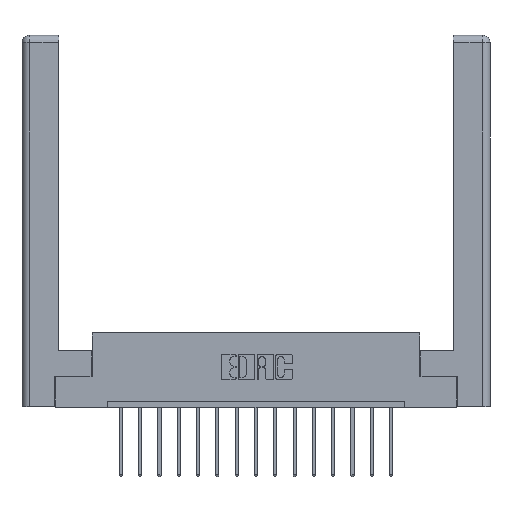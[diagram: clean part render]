
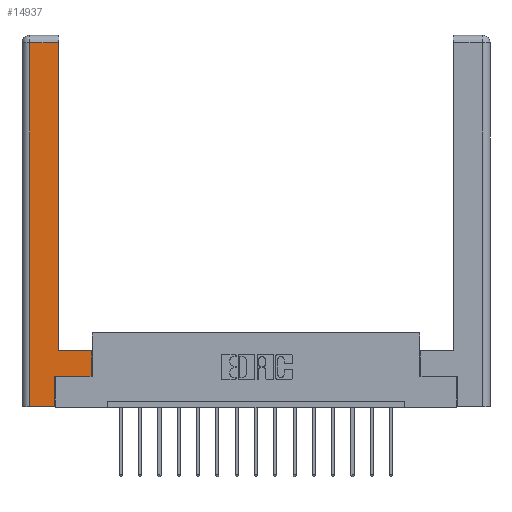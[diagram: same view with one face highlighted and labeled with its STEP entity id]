
A CAD part, top view. The second image highlights one B-rep face of the part: STEP entity #14937.
In plain terms, the highlighted planar face has unit normal (0, 0, 1).
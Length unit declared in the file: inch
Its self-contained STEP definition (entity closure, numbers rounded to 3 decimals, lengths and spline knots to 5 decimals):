
#40 = VERTEX_POINT ( 'NONE', #4370 ) ;
#230 = LINE ( 'NONE', #13542, #3370 ) ;
#260 = ORIENTED_EDGE ( 'NONE', *, *, #15609, .T. ) ;
#783 = LINE ( 'NONE', #4353, #16887 ) ;
#900 = ORIENTED_EDGE ( 'NONE', *, *, #16479, .T. ) ;
#948 = CARTESIAN_POINT ( 'NONE',  ( 0., 0., 0. ) ) ;
#1751 = CARTESIAN_POINT ( 'NONE',  ( 0.565, 0.245, 0. ) ) ;
#1812 = CARTESIAN_POINT ( 'NONE',  ( 0.265, 0., 0. ) ) ;
#1978 = EDGE_CURVE ( 'NONE', #3617, #40, #2617, .T. ) ;
#2028 = DIRECTION ( 'NONE',  ( 0., 1., 0. ) ) ;
#2090 = VECTOR ( 'NONE', #13930, 39.37008 ) ;
#2292 = DIRECTION ( 'NONE',  ( -1., 0., 0. ) ) ;
#2515 = EDGE_CURVE ( 'NONE', #40, #6426, #5621, .T. ) ;
#2617 = LINE ( 'NONE', #8332, #12903 ) ;
#2991 = VERTEX_POINT ( 'NONE', #9175 ) ;
#3073 = DIRECTION ( 'NONE',  ( 1., 0., 0. ) ) ;
#3102 = DIRECTION ( 'NONE',  ( 0., -1., 0. ) ) ;
#3370 = VECTOR ( 'NONE', #14825, 39.37008 ) ;
#3522 = LINE ( 'NONE', #4720, #11499 ) ;
#3585 = PLANE ( 'NONE',  #16337 ) ;
#3617 = VERTEX_POINT ( 'NONE', #6560 ) ;
#3677 = EDGE_CURVE ( 'NONE', #7343, #13617, #783, .T. ) ;
#4034 = EDGE_CURVE ( 'NONE', #16608, #12767, #5981, .T. ) ;
#4199 = ORIENTED_EDGE ( 'NONE', *, *, #3677, .T. ) ;
#4353 = CARTESIAN_POINT ( 'NONE',  ( 0.265, 0., 0. ) ) ;
#4370 = CARTESIAN_POINT ( 'NONE',  ( 0.295, 2.94, 0. ) ) ;
#4395 = CARTESIAN_POINT ( 'NONE',  ( 0.565, 0.245, 0. ) ) ;
#4586 = CARTESIAN_POINT ( 'NONE',  ( 0.0615, 0., 0. ) ) ;
#4720 = CARTESIAN_POINT ( 'NONE',  ( 0.265, 0.245, 0. ) ) ;
#5621 = LINE ( 'NONE', #12556, #2090 ) ;
#5915 = CARTESIAN_POINT ( 'NONE',  ( 0.0615, 0., 0. ) ) ;
#5981 = LINE ( 'NONE', #14539, #14629 ) ;
#6426 = VERTEX_POINT ( 'NONE', #10384 ) ;
#6515 = LINE ( 'NONE', #1751, #16730 ) ;
#6560 = CARTESIAN_POINT ( 'NONE',  ( 0.295, 0.45, 0. ) ) ;
#6942 = FACE_OUTER_BOUND ( 'NONE', #14401, .T. ) ;
#7056 = DIRECTION ( 'NONE',  ( 1., 0., 0. ) ) ;
#7093 = DIRECTION ( 'NONE',  ( 0., 1., 0. ) ) ;
#7343 = VERTEX_POINT ( 'NONE', #5915 ) ;
#7631 = ORIENTED_EDGE ( 'NONE', *, *, #7896, .T. ) ;
#7896 = EDGE_CURVE ( 'NONE', #12767, #3617, #230, .T. ) ;
#8332 = CARTESIAN_POINT ( 'NONE',  ( 0.295, 3., 0. ) ) ;
#8347 = LINE ( 'NONE', #4586, #14660 ) ;
#9175 = CARTESIAN_POINT ( 'NONE',  ( 0.265, 0.245, 0. ) ) ;
#10384 = CARTESIAN_POINT ( 'NONE',  ( 0.0615, 2.94, 0. ) ) ;
#10911 = CARTESIAN_POINT ( 'NONE',  ( 0.565, 0.45, 0. ) ) ;
#11499 = VECTOR ( 'NONE', #2028, 39.37008 ) ;
#12556 = CARTESIAN_POINT ( 'NONE',  ( 0.0615, 2.94, 0. ) ) ;
#12767 = VERTEX_POINT ( 'NONE', #10911 ) ;
#12903 = VECTOR ( 'NONE', #7093, 39.37008 ) ;
#13542 = CARTESIAN_POINT ( 'NONE',  ( 0.295, 0.45, 0. ) ) ;
#13617 = VERTEX_POINT ( 'NONE', #1812 ) ;
#13930 = DIRECTION ( 'NONE',  ( -1., 0., 0. ) ) ;
#14401 = EDGE_LOOP ( 'NONE', ( #17290, #16753, #15548, #4199, #900, #260, #14487, #7631 ) ) ;
#14487 = ORIENTED_EDGE ( 'NONE', *, *, #4034, .T. ) ;
#14539 = CARTESIAN_POINT ( 'NONE',  ( 0.565, 0.45, 0. ) ) ;
#14629 = VECTOR ( 'NONE', #15201, 39.37008 ) ;
#14660 = VECTOR ( 'NONE', #3102, 39.37008 ) ;
#14825 = DIRECTION ( 'NONE',  ( -1., 0., 0. ) ) ;
#14937 = ADVANCED_FACE ( 'NONE', ( #6942 ), #3585, .F. ) ;
#15201 = DIRECTION ( 'NONE',  ( 0., 1., 0. ) ) ;
#15548 = ORIENTED_EDGE ( 'NONE', *, *, #16332, .T. ) ;
#15609 = EDGE_CURVE ( 'NONE', #2991, #16608, #6515, .T. ) ;
#15734 = DIRECTION ( 'NONE',  ( 0., 0., -1. ) ) ;
#16332 = EDGE_CURVE ( 'NONE', #6426, #7343, #8347, .T. ) ;
#16337 = AXIS2_PLACEMENT_3D ( 'NONE', #948, #15734, #2292 ) ;
#16479 = EDGE_CURVE ( 'NONE', #13617, #2991, #3522, .T. ) ;
#16608 = VERTEX_POINT ( 'NONE', #4395 ) ;
#16730 = VECTOR ( 'NONE', #3073, 39.37008 ) ;
#16753 = ORIENTED_EDGE ( 'NONE', *, *, #2515, .T. ) ;
#16887 = VECTOR ( 'NONE', #7056, 39.37008 ) ;
#17290 = ORIENTED_EDGE ( 'NONE', *, *, #1978, .T. ) ;
